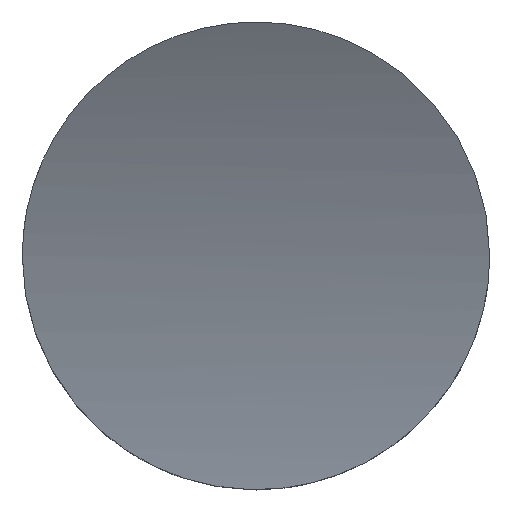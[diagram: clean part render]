
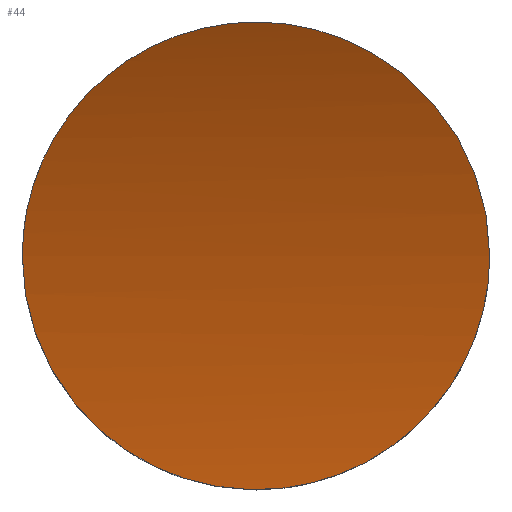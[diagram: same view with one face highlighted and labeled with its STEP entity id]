
A CAD part, top view. The second image highlights one B-rep face of the part: STEP entity #44.
In plain terms, the highlighted cylindrical face has radius 19.05 mm (diameter 38.1 mm), a partial arc.
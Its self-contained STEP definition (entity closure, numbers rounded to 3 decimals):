
#2 = ORIENTED_EDGE ( 'NONE', *, *, #175, .T. ) ;
#6 = CYLINDRICAL_SURFACE ( 'NONE', #42, 19.05 ) ;
#8 = CARTESIAN_POINT ( 'NONE',  ( -55.693, -30.677, 2.477 ) ) ;
#9 = CARTESIAN_POINT ( 'NONE',  ( -57.649, -31.509, 2.288 ) ) ;
#10 = DIRECTION ( 'NONE',  ( -1., 0., 0. ) ) ;
#12 = CARTESIAN_POINT ( 'NONE',  ( -46.362, -35.333, 20.95 ) ) ;
#13 = CARTESIAN_POINT ( 'NONE',  ( -57.411, -25.058, 4.909 ) ) ;
#15 = B_SPLINE_CURVE_WITH_KNOTS ( 'NONE', 3,
 ( #179, #84, #123, #109, #190, #28, #157, #78, #174, #77, #173, #89, #90, #186, #106, #9, #122, #22, #135, #45, #151, #24, #8, #46, #21, #150, #133, #121, #62, #88, #104, #43 ),
 .UNSPECIFIED., .F., .F.,
 ( 4, 2, 2, 2, 2, 2, 2, 2, 2, 2, 2, 2, 2, 2, 2, 4 ),
 ( 0.016, 0.017, 0.017, 0.018, 0.019, 0.019, 0.02, 0.021, 0.022, 0.022, 0.023, 0.024, 0.024, 0.025, 0.026, 0.026 ),
 .UNSPECIFIED. ) ;
#16 = CARTESIAN_POINT ( 'NONE',  ( -60.799, -26.872, 3.881 ) ) ;
#21 = CARTESIAN_POINT ( 'NONE',  ( -55.265, -30.205, 2.602 ) ) ;
#22 = CARTESIAN_POINT ( 'NONE',  ( -57.01, -31.401, 2.31 ) ) ;
#24 = CARTESIAN_POINT ( 'NONE',  ( -55.859, -30.818, 2.443 ) ) ;
#27 = B_SPLINE_CURVE_WITH_KNOTS ( 'NONE', 3,
 ( #143, #80, #49, #33, #94, #187, #116, #64, #159, #55, #142, #169, #71, #13, #125, #30, #138, #68, #52, #153, #164, #82, #178, #113, #96, #192, #16, #126, #32, #139, #53, #155 ),
 .UNSPECIFIED., .F., .F.,
 ( 4, 2, 2, 2, 2, 2, 2, 2, 2, 2, 2, 2, 2, 2, 2, 4 ),
 ( 0.005, 0.006, 0.007, 0.007, 0.008, 0.009, 0.01, 0.011, 0.011, 0.012, 0.013, 0.013, 0.014, 0.015, 0.015, 0.016 ),
 .UNSPECIFIED. ) ;
#28 = CARTESIAN_POINT ( 'NONE',  ( -60.803, -29.662, 2.763 ) ) ;
#30 = CARTESIAN_POINT ( 'NONE',  ( -58.088, -25.032, 4.925 ) ) ;
#32 = CARTESIAN_POINT ( 'NONE',  ( -61.01, -27.449, 3.607 ) ) ;
#33 = CARTESIAN_POINT ( 'NONE',  ( -54.732, -27.45, 3.606 ) ) ;
#37 = VERTEX_POINT ( 'NONE', #91 ) ;
#42 = AXIS2_PLACEMENT_3D ( 'NONE', #12, #10, #111 ) ;
#43 = CARTESIAN_POINT ( 'NONE',  ( -54.633, -28.271, 3.257 ) ) ;
#44 = ADVANCED_FACE ( 'NONE', ( #50 ), #6, .F. ) ;
#45 = CARTESIAN_POINT ( 'NONE',  ( -56.402, -31.165, 2.361 ) ) ;
#46 = CARTESIAN_POINT ( 'NONE',  ( -55.397, -30.372, 2.557 ) ) ;
#49 = CARTESIAN_POINT ( 'NONE',  ( -54.653, -27.853, 3.429 ) ) ;
#50 = FACE_OUTER_BOUND ( 'NONE', #79, .T. ) ;
#52 = CARTESIAN_POINT ( 'NONE',  ( -58.962, -25.214, 4.81 ) ) ;
#53 = CARTESIAN_POINT ( 'NONE',  ( -61.11, -28.063, 3.341 ) ) ;
#55 = CARTESIAN_POINT ( 'NONE',  ( -55.822, -25.729, 4.495 ) ) ;
#59 = VERTEX_POINT ( 'NONE', #128 ) ;
#62 = CARTESIAN_POINT ( 'NONE',  ( -54.728, -29.076, 2.956 ) ) ;
#64 = CARTESIAN_POINT ( 'NONE',  ( -55.26, -26.345, 4.153 ) ) ;
#68 = CARTESIAN_POINT ( 'NONE',  ( -58.75, -25.146, 4.853 ) ) ;
#71 = CARTESIAN_POINT ( 'NONE',  ( -56.979, -25.15, 4.85 ) ) ;
#77 = CARTESIAN_POINT ( 'NONE',  ( -60.049, -30.677, 2.477 ) ) ;
#78 = CARTESIAN_POINT ( 'NONE',  ( -60.48, -30.202, 2.603 ) ) ;
#79 = EDGE_LOOP ( 'NONE', ( #2, #132 ) ) ;
#80 = CARTESIAN_POINT ( 'NONE',  ( -54.633, -28.062, 3.341 ) ) ;
#82 = CARTESIAN_POINT ( 'NONE',  ( -59.902, -25.739, 4.492 ) ) ;
#84 = CARTESIAN_POINT ( 'NONE',  ( -61.11, -28.473, 3.177 ) ) ;
#88 = CARTESIAN_POINT ( 'NONE',  ( -54.651, -28.674, 3.101 ) ) ;
#89 = CARTESIAN_POINT ( 'NONE',  ( -59.53, -31.061, 2.385 ) ) ;
#90 = CARTESIAN_POINT ( 'NONE',  ( -59.338, -31.166, 2.361 ) ) ;
#91 = CARTESIAN_POINT ( 'NONE',  ( -54.633, -28.271, 3.257 ) ) ;
#94 = CARTESIAN_POINT ( 'NONE',  ( -54.79, -27.254, 3.697 ) ) ;
#96 = CARTESIAN_POINT ( 'NONE',  ( -60.481, -26.342, 4.154 ) ) ;
#104 = CARTESIAN_POINT ( 'NONE',  ( -54.633, -28.473, 3.177 ) ) ;
#106 = CARTESIAN_POINT ( 'NONE',  ( -58.306, -31.51, 2.288 ) ) ;
#109 = CARTESIAN_POINT ( 'NONE',  ( -61.015, -29.074, 2.956 ) ) ;
#111 = DIRECTION ( 'NONE',  ( 0., 0.995, -0.105 ) ) ;
#113 = CARTESIAN_POINT ( 'NONE',  ( -60.353, -26.18, 4.242 ) ) ;
#116 = CARTESIAN_POINT ( 'NONE',  ( -55.038, -26.689, 3.973 ) ) ;
#121 = CARTESIAN_POINT ( 'NONE',  ( -54.786, -29.277, 2.887 ) ) ;
#122 = CARTESIAN_POINT ( 'NONE',  ( -57.434, -31.487, 2.292 ) ) ;
#123 = CARTESIAN_POINT ( 'NONE',  ( -61.091, -28.674, 3.101 ) ) ;
#125 = CARTESIAN_POINT ( 'NONE',  ( -57.638, -25.033, 4.925 ) ) ;
#126 = CARTESIAN_POINT ( 'NONE',  ( -60.952, -27.253, 3.697 ) ) ;
#128 = CARTESIAN_POINT ( 'NONE',  ( -61.11, -28.271, 3.257 ) ) ;
#132 = ORIENTED_EDGE ( 'NONE', *, *, #141, .T. ) ;
#133 = CARTESIAN_POINT ( 'NONE',  ( -54.939, -29.662, 2.763 ) ) ;
#135 = CARTESIAN_POINT ( 'NONE',  ( -56.8, -31.335, 2.324 ) ) ;
#138 = CARTESIAN_POINT ( 'NONE',  ( -58.31, -25.055, 4.911 ) ) ;
#139 = CARTESIAN_POINT ( 'NONE',  ( -61.089, -27.853, 3.429 ) ) ;
#141 = EDGE_CURVE ( 'NONE', #37, #59, #27, .T. ) ;
#142 = CARTESIAN_POINT ( 'NONE',  ( -56.165, -25.483, 4.643 ) ) ;
#143 = CARTESIAN_POINT ( 'NONE',  ( -54.633, -28.271, 3.257 ) ) ;
#150 = CARTESIAN_POINT ( 'NONE',  ( -55.035, -29.848, 2.706 ) ) ;
#151 = CARTESIAN_POINT ( 'NONE',  ( -56.214, -31.062, 2.385 ) ) ;
#153 = CARTESIAN_POINT ( 'NONE',  ( -59.362, -25.388, 4.702 ) ) ;
#155 = CARTESIAN_POINT ( 'NONE',  ( -61.11, -28.271, 3.257 ) ) ;
#157 = CARTESIAN_POINT ( 'NONE',  ( -60.708, -29.848, 2.706 ) ) ;
#159 = CARTESIAN_POINT ( 'NONE',  ( -55.387, -26.183, 4.241 ) ) ;
#164 = CARTESIAN_POINT ( 'NONE',  ( -59.553, -25.495, 4.636 ) ) ;
#169 = CARTESIAN_POINT ( 'NONE',  ( -56.77, -25.218, 4.807 ) ) ;
#173 = CARTESIAN_POINT ( 'NONE',  ( -59.886, -30.816, 2.443 ) ) ;
#174 = CARTESIAN_POINT ( 'NONE',  ( -60.345, -30.371, 2.557 ) ) ;
#175 = EDGE_CURVE ( 'NONE', #59, #37, #15, .T. ) ;
#178 = CARTESIAN_POINT ( 'NONE',  ( -60.061, -25.876, 4.412 ) ) ;
#179 = CARTESIAN_POINT ( 'NONE',  ( -61.11, -28.271, 3.257 ) ) ;
#186 = CARTESIAN_POINT ( 'NONE',  ( -58.743, -31.42, 2.306 ) ) ;
#187 = CARTESIAN_POINT ( 'NONE',  ( -54.943, -26.872, 3.881 ) ) ;
#190 = CARTESIAN_POINT ( 'NONE',  ( -60.957, -29.276, 2.888 ) ) ;
#192 = CARTESIAN_POINT ( 'NONE',  ( -60.703, -26.687, 3.974 ) ) ;
